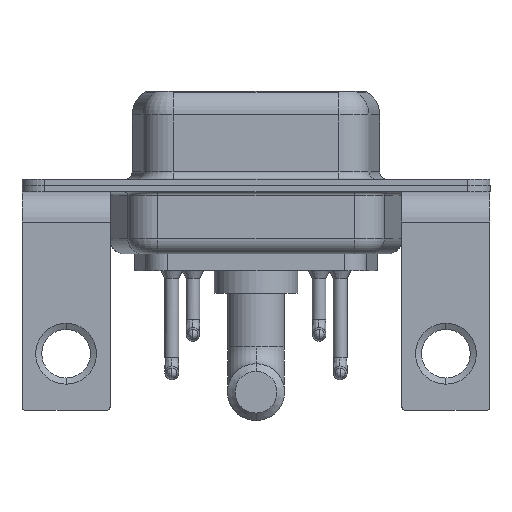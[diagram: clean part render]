
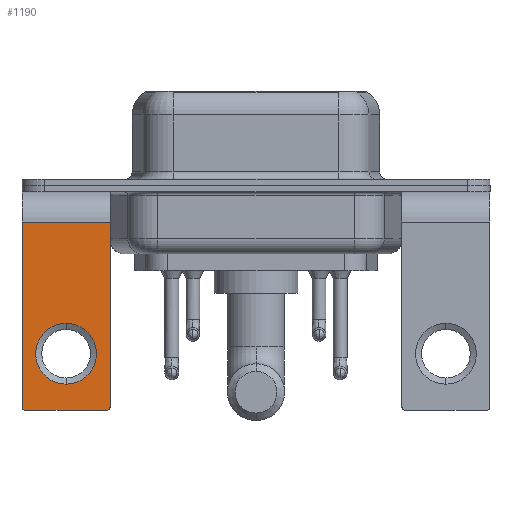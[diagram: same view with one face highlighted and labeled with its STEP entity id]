
A CAD part, front view. The second image highlights one B-rep face of the part: STEP entity #1190.
In plain terms, the highlighted planar face has unit normal (0, -1, 0).
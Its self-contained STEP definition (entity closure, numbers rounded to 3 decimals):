
#187 = EDGE_CURVE ( 'NONE', #5759, #15010, #4981, .T. ) ;
#555 = EDGE_LOOP ( 'NONE', ( #2879, #10555, #7607, #1641, #4521, #8586 ) ) ;
#609 = DIRECTION ( 'NONE',  ( 0., 0., 1. ) ) ;
#799 = DIRECTION ( 'NONE',  ( -1., 0., 0. ) ) ;
#857 = DIRECTION ( 'NONE',  ( 0., -1., 0. ) ) ;
#1190 = ADVANCED_FACE ( 'NONE', ( #4441, #11337 ), #3159, .F. ) ;
#1558 = EDGE_CURVE ( 'NONE', #15010, #5759, #12445, .T. ) ;
#1562 = VERTEX_POINT ( 'NONE', #4080 ) ;
#1641 = ORIENTED_EDGE ( 'NONE', *, *, #15615, .T. ) ;
#1695 = EDGE_CURVE ( 'NONE', #4184, #4005, #15119, .T. ) ;
#1926 = EDGE_CURVE ( 'NONE', #2965, #13337, #4059, .T. ) ;
#2879 = ORIENTED_EDGE ( 'NONE', *, *, #10497, .T. ) ;
#2965 = VERTEX_POINT ( 'NONE', #6673 ) ;
#3159 = PLANE ( 'NONE',  #14355 ) ;
#3973 = DIRECTION ( 'NONE',  ( 0., 0., -1. ) ) ;
#4005 = VERTEX_POINT ( 'NONE', #11707 ) ;
#4059 = LINE ( 'NONE', #9303, #10235 ) ;
#4080 = CARTESIAN_POINT ( 'NONE',  ( -2.9, -6.25, -14.55 ) ) ;
#4184 = VERTEX_POINT ( 'NONE', #9795 ) ;
#4239 = CIRCLE ( 'NONE', #9751, 0.25 ) ;
#4441 = FACE_BOUND ( 'NONE', #10621, .T. ) ;
#4491 = EDGE_CURVE ( 'NONE', #1562, #4005, #4239, .T. ) ;
#4521 = ORIENTED_EDGE ( 'NONE', *, *, #1926, .F. ) ;
#4566 = ORIENTED_EDGE ( 'NONE', *, *, #1558, .T. ) ;
#4964 = CIRCLE ( 'NONE', #15997, 0.25 ) ;
#4981 = CIRCLE ( 'NONE', #14645, 2. ) ;
#5440 = LINE ( 'NONE', #10858, #5698 ) ;
#5641 = CARTESIAN_POINT ( 'NONE',  ( 0., -6.25, -11.07 ) ) ;
#5698 = VECTOR ( 'NONE', #10679, 1000. ) ;
#5759 = VERTEX_POINT ( 'NONE', #14532 ) ;
#6122 = CARTESIAN_POINT ( 'NONE',  ( -2.9, -6.25, -2.4 ) ) ;
#6167 = DIRECTION ( 'NONE',  ( 0., 0., 1. ) ) ;
#6360 = CARTESIAN_POINT ( 'NONE',  ( -2.9, -6.25, -2.4 ) ) ;
#6673 = CARTESIAN_POINT ( 'NONE',  ( 2.9, -6.25, -2.4 ) ) ;
#6741 = DIRECTION ( 'NONE',  ( 0., 0., 1. ) ) ;
#6757 = CARTESIAN_POINT ( 'NONE',  ( 0., -6.25, -13.07 ) ) ;
#7607 = ORIENTED_EDGE ( 'NONE', *, *, #1695, .F. ) ;
#7951 = CARTESIAN_POINT ( 'NONE',  ( -2.65, -6.25, -14.55 ) ) ;
#8138 = DIRECTION ( 'NONE',  ( 0., 0., 1. ) ) ;
#8172 = EDGE_CURVE ( 'NONE', #2965, #14336, #5440, .T. ) ;
#8569 = VECTOR ( 'NONE', #799, 1000. ) ;
#8586 = ORIENTED_EDGE ( 'NONE', *, *, #8172, .T. ) ;
#9246 = DIRECTION ( 'NONE',  ( 0., 0., 1. ) ) ;
#9303 = CARTESIAN_POINT ( 'NONE',  ( 2.9, -6.25, -2.4 ) ) ;
#9751 = AXIS2_PLACEMENT_3D ( 'NONE', #7951, #11857, #9246 ) ;
#9795 = CARTESIAN_POINT ( 'NONE',  ( 2.65, -6.25, -14.8 ) ) ;
#10235 = VECTOR ( 'NONE', #3973, 1000. ) ;
#10497 = EDGE_CURVE ( 'NONE', #14336, #1562, #15585, .T. ) ;
#10555 = ORIENTED_EDGE ( 'NONE', *, *, #4491, .T. ) ;
#10621 = EDGE_LOOP ( 'NONE', ( #4566, #11075 ) ) ;
#10679 = DIRECTION ( 'NONE',  ( -1., 0., 0. ) ) ;
#10796 = DIRECTION ( 'NONE',  ( 0., 1., 0. ) ) ;
#10858 = CARTESIAN_POINT ( 'NONE',  ( 2.9, -6.25, -2.4 ) ) ;
#11075 = ORIENTED_EDGE ( 'NONE', *, *, #187, .T. ) ;
#11337 = FACE_OUTER_BOUND ( 'NONE', #555, .T. ) ;
#11707 = CARTESIAN_POINT ( 'NONE',  ( -2.65, -6.25, -14.8 ) ) ;
#11857 = DIRECTION ( 'NONE',  ( 0., -1., 0. ) ) ;
#12313 = DIRECTION ( 'NONE',  ( 0., 1., 0. ) ) ;
#12445 = CIRCLE ( 'NONE', #16031, 2. ) ;
#12484 = CARTESIAN_POINT ( 'NONE',  ( 2.9, -6.25, -2.4 ) ) ;
#13191 = CARTESIAN_POINT ( 'NONE',  ( 2.9, -6.25, -14.55 ) ) ;
#13337 = VERTEX_POINT ( 'NONE', #13191 ) ;
#13525 = CARTESIAN_POINT ( 'NONE',  ( 0., -6.25, -11.07 ) ) ;
#13740 = CARTESIAN_POINT ( 'NONE',  ( 2.9, -6.25, -14.8 ) ) ;
#13917 = VECTOR ( 'NONE', #15256, 1000. ) ;
#13969 = CARTESIAN_POINT ( 'NONE',  ( 2.65, -6.25, -14.55 ) ) ;
#14336 = VERTEX_POINT ( 'NONE', #6122 ) ;
#14355 = AXIS2_PLACEMENT_3D ( 'NONE', #12484, #16616, #6167 ) ;
#14532 = CARTESIAN_POINT ( 'NONE',  ( 0., -6.25, -9.07 ) ) ;
#14645 = AXIS2_PLACEMENT_3D ( 'NONE', #13525, #12313, #8138 ) ;
#15010 = VERTEX_POINT ( 'NONE', #6757 ) ;
#15119 = LINE ( 'NONE', #13740, #8569 ) ;
#15256 = DIRECTION ( 'NONE',  ( 0., 0., -1. ) ) ;
#15585 = LINE ( 'NONE', #6360, #13917 ) ;
#15615 = EDGE_CURVE ( 'NONE', #4184, #13337, #4964, .T. ) ;
#15997 = AXIS2_PLACEMENT_3D ( 'NONE', #13969, #857, #609 ) ;
#16031 = AXIS2_PLACEMENT_3D ( 'NONE', #5641, #10796, #6741 ) ;
#16616 = DIRECTION ( 'NONE',  ( 0., 1., 0. ) ) ;
